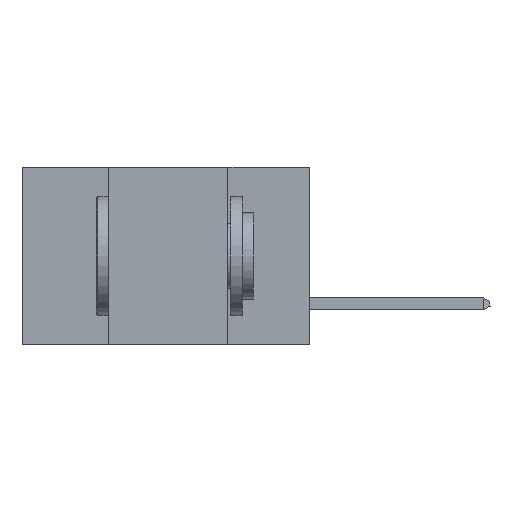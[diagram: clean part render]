
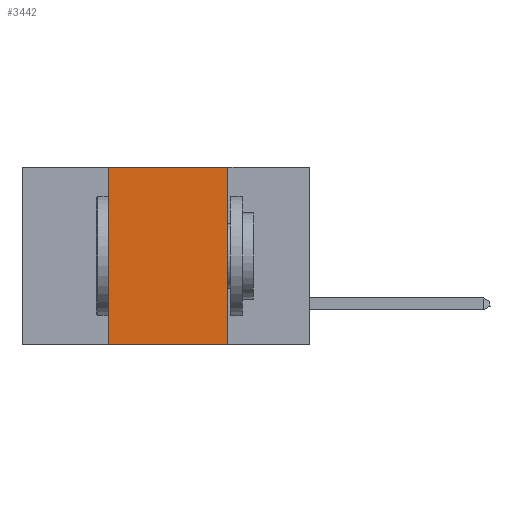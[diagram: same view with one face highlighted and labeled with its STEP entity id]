
A CAD part, left-side view. The second image highlights one B-rep face of the part: STEP entity #3442.
In plain terms, the highlighted planar face has unit normal (-1, 0, 0).
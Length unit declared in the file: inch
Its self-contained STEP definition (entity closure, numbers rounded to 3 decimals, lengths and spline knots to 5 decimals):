
#610 = CARTESIAN_POINT ( 'NONE',  ( 0., 0.42, -0.37 ) ) ;
#842 = VECTOR ( 'NONE', #10510, 39.37008 ) ;
#1249 = PLANE ( 'NONE',  #13713 ) ;
#1571 = VECTOR ( 'NONE', #10689, 39.37008 ) ;
#2048 = LINE ( 'NONE', #10374, #7631 ) ;
#2879 = CARTESIAN_POINT ( 'NONE',  ( 0., 0.17, 0. ) ) ;
#2974 = ORIENTED_EDGE ( 'NONE', *, *, #21515, .F. ) ;
#3348 = CARTESIAN_POINT ( 'NONE',  ( 0., 0.42, 0. ) ) ;
#3442 = ADVANCED_FACE ( 'NONE', ( #12383 ), #1249, .F. ) ;
#3531 = ORIENTED_EDGE ( 'NONE', *, *, #4870, .F. ) ;
#4870 = EDGE_CURVE ( 'NONE', #7903, #23784, #5845, .T. ) ;
#5651 = VERTEX_POINT ( 'NONE', #610 ) ;
#5845 = LINE ( 'NONE', #23148, #842 ) ;
#5996 = LINE ( 'NONE', #2879, #11310 ) ;
#6307 = EDGE_LOOP ( 'NONE', ( #22633, #3531, #2974, #6503 ) ) ;
#6405 = CARTESIAN_POINT ( 'NONE',  ( 0., 0.17, -0.37 ) ) ;
#6503 = ORIENTED_EDGE ( 'NONE', *, *, #8759, .T. ) ;
#7583 = CARTESIAN_POINT ( 'NONE',  ( 0., 0.6, 0. ) ) ;
#7631 = VECTOR ( 'NONE', #23276, 39.37008 ) ;
#7903 = VERTEX_POINT ( 'NONE', #3348 ) ;
#8759 = EDGE_CURVE ( 'NONE', #5651, #21127, #11584, .T. ) ;
#10374 = CARTESIAN_POINT ( 'NONE',  ( 0., 0.42, 0. ) ) ;
#10510 = DIRECTION ( 'NONE',  ( 0., -1., 0. ) ) ;
#10689 = DIRECTION ( 'NONE',  ( 0., -1., 0. ) ) ;
#11206 = DIRECTION ( 'NONE',  ( 0., 0., -1. ) ) ;
#11310 = VECTOR ( 'NONE', #17851, 39.37008 ) ;
#11584 = LINE ( 'NONE', #16536, #1571 ) ;
#12383 = FACE_OUTER_BOUND ( 'NONE', #6307, .T. ) ;
#13713 = AXIS2_PLACEMENT_3D ( 'NONE', #7583, #14965, #11206 ) ;
#13930 = CARTESIAN_POINT ( 'NONE',  ( 0., 0.17, 0. ) ) ;
#14078 = EDGE_CURVE ( 'NONE', #23784, #21127, #5996, .T. ) ;
#14965 = DIRECTION ( 'NONE',  ( 1., 0., 0. ) ) ;
#16536 = CARTESIAN_POINT ( 'NONE',  ( 0., 0.6, -0.37 ) ) ;
#17851 = DIRECTION ( 'NONE',  ( 0., 0., -1. ) ) ;
#21127 = VERTEX_POINT ( 'NONE', #6405 ) ;
#21515 = EDGE_CURVE ( 'NONE', #5651, #7903, #2048, .T. ) ;
#22633 = ORIENTED_EDGE ( 'NONE', *, *, #14078, .F. ) ;
#23148 = CARTESIAN_POINT ( 'NONE',  ( 0., 0.6, 0. ) ) ;
#23276 = DIRECTION ( 'NONE',  ( 0., 0., 1. ) ) ;
#23784 = VERTEX_POINT ( 'NONE', #13930 ) ;
